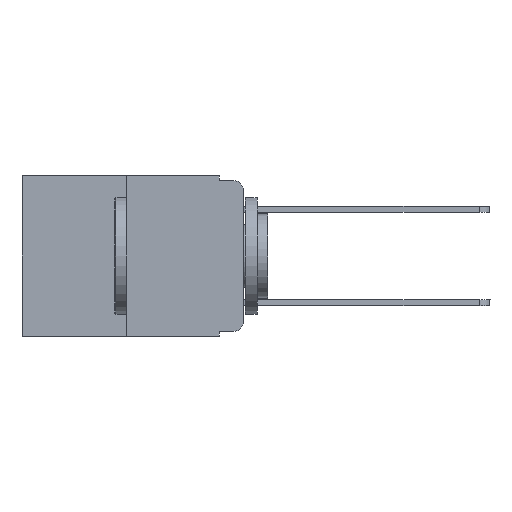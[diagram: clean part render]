
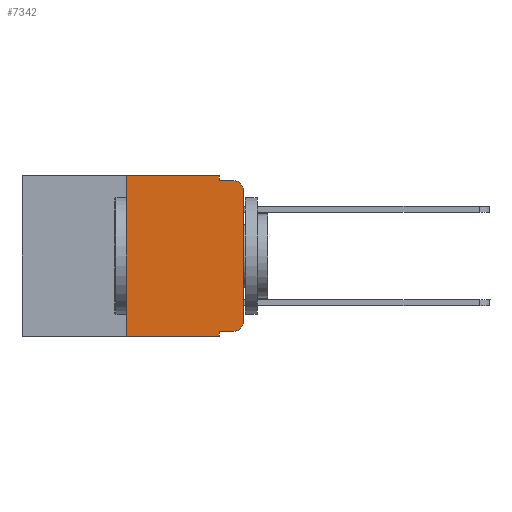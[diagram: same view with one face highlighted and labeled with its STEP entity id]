
A CAD part, left-side view. The second image highlights one B-rep face of the part: STEP entity #7342.
In plain terms, the highlighted planar face has unit normal (-1, 0, 0).
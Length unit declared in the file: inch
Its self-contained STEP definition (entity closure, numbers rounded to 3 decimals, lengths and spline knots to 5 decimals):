
#190 = CARTESIAN_POINT ( 'NONE',  ( 0., 0.02, -0.333 ) ) ;
#221 = AXIS2_PLACEMENT_3D ( 'NONE', #11391, #11540, #12854 ) ;
#326 = EDGE_CURVE ( 'NONE', #5018, #15026, #14338, .T. ) ;
#525 = DIRECTION ( 'NONE',  ( 0., 0., -1. ) ) ;
#874 = ORIENTED_EDGE ( 'NONE', *, *, #3937, .F. ) ;
#969 = ORIENTED_EDGE ( 'NONE', *, *, #7235, .T. ) ;
#1090 = CARTESIAN_POINT ( 'NONE',  ( 0., 0.051, -0.333 ) ) ;
#1106 = VECTOR ( 'NONE', #8067, 39.37008 ) ;
#1108 = ORIENTED_EDGE ( 'NONE', *, *, #9975, .T. ) ;
#1454 = EDGE_CURVE ( 'NONE', #6162, #4682, #5927, .T. ) ;
#1470 = EDGE_CURVE ( 'NONE', #2970, #7598, #14692, .T. ) ;
#1825 = CARTESIAN_POINT ( 'NONE',  ( 0., 0.051, 0. ) ) ;
#1894 = CARTESIAN_POINT ( 'NONE',  ( 0., 0., -0.313 ) ) ;
#2095 = LINE ( 'NONE', #7266, #9071 ) ;
#2244 = CIRCLE ( 'NONE', #221, 0.02 ) ;
#2262 = VECTOR ( 'NONE', #8314, 39.37008 ) ;
#2296 = EDGE_CURVE ( 'NONE', #5897, #6148, #2095, .T. ) ;
#2674 = ORIENTED_EDGE ( 'NONE', *, *, #8245, .F. ) ;
#2822 = LINE ( 'NONE', #1825, #8971 ) ;
#2970 = VERTEX_POINT ( 'NONE', #1894 ) ;
#2978 = ORIENTED_EDGE ( 'NONE', *, *, #8376, .F. ) ;
#3019 = PLANE ( 'NONE',  #7174 ) ;
#3064 = CARTESIAN_POINT ( 'NONE',  ( 0., 0.25, 0. ) ) ;
#3138 = VECTOR ( 'NONE', #14092, 39.37008 ) ;
#3145 = LINE ( 'NONE', #3064, #1106 ) ;
#3376 = CARTESIAN_POINT ( 'NONE',  ( 0., 0.051, -0.01 ) ) ;
#3489 = CARTESIAN_POINT ( 'NONE',  ( 0., 0., -0.03 ) ) ;
#3937 = EDGE_CURVE ( 'NONE', #8508, #12610, #4305, .T. ) ;
#4182 = ORIENTED_EDGE ( 'NONE', *, *, #326, .F. ) ;
#4305 = LINE ( 'NONE', #7858, #4400 ) ;
#4400 = VECTOR ( 'NONE', #14241, 39.37008 ) ;
#4682 = VERTEX_POINT ( 'NONE', #190 ) ;
#4805 = LINE ( 'NONE', #5873, #14015 ) ;
#4970 = DIRECTION ( 'NONE',  ( 0., -1., 0. ) ) ;
#5018 = VERTEX_POINT ( 'NONE', #10090 ) ;
#5476 = DIRECTION ( 'NONE',  ( 1., 0., 0. ) ) ;
#5873 = CARTESIAN_POINT ( 'NONE',  ( 0., 0.051, 0. ) ) ;
#5897 = VERTEX_POINT ( 'NONE', #8848 ) ;
#5927 = LINE ( 'NONE', #1090, #2262 ) ;
#6086 = AXIS2_PLACEMENT_3D ( 'NONE', #7183, #8176, #8341 ) ;
#6148 = VERTEX_POINT ( 'NONE', #8497 ) ;
#6162 = VERTEX_POINT ( 'NONE', #8583 ) ;
#6395 = CARTESIAN_POINT ( 'NONE',  ( 0., 0.02, -0.01 ) ) ;
#7174 = AXIS2_PLACEMENT_3D ( 'NONE', #15721, #5476, #9412 ) ;
#7183 = CARTESIAN_POINT ( 'NONE',  ( 0., 0.02, -0.03 ) ) ;
#7235 = EDGE_CURVE ( 'NONE', #4682, #2970, #2244, .T. ) ;
#7266 = CARTESIAN_POINT ( 'NONE',  ( 0., 0.473, -0.343 ) ) ;
#7342 = ADVANCED_FACE ( 'NONE', ( #13242 ), #3019, .F. ) ;
#7367 = ORIENTED_EDGE ( 'NONE', *, *, #1470, .T. ) ;
#7380 = CARTESIAN_POINT ( 'NONE',  ( 0., 0.051, 0. ) ) ;
#7598 = VERTEX_POINT ( 'NONE', #3489 ) ;
#7858 = CARTESIAN_POINT ( 'NONE',  ( 0., 0.051, -0.01 ) ) ;
#8011 = EDGE_LOOP ( 'NONE', ( #7367, #1108, #874, #2674, #4182, #2978, #10095, #13041, #8212, #969 ) ) ;
#8067 = DIRECTION ( 'NONE',  ( 0., 0., 1. ) ) ;
#8176 = DIRECTION ( 'NONE',  ( -1., 0., 0. ) ) ;
#8212 = ORIENTED_EDGE ( 'NONE', *, *, #1454, .T. ) ;
#8245 = EDGE_CURVE ( 'NONE', #15026, #8508, #2822, .T. ) ;
#8314 = DIRECTION ( 'NONE',  ( 0., -1., 0. ) ) ;
#8341 = DIRECTION ( 'NONE',  ( 0., 0., -1. ) ) ;
#8376 = EDGE_CURVE ( 'NONE', #5897, #5018, #3145, .T. ) ;
#8420 = DIRECTION ( 'NONE',  ( 0., 0., -1. ) ) ;
#8497 = CARTESIAN_POINT ( 'NONE',  ( 0., 0.051, -0.343 ) ) ;
#8508 = VERTEX_POINT ( 'NONE', #3376 ) ;
#8583 = CARTESIAN_POINT ( 'NONE',  ( 0., 0.051, -0.333 ) ) ;
#8848 = CARTESIAN_POINT ( 'NONE',  ( 0., 0.25, -0.343 ) ) ;
#8971 = VECTOR ( 'NONE', #525, 39.37008 ) ;
#9071 = VECTOR ( 'NONE', #4970, 39.37008 ) ;
#9412 = DIRECTION ( 'NONE',  ( 0., 0., -1. ) ) ;
#9975 = EDGE_CURVE ( 'NONE', #7598, #12610, #15771, .T. ) ;
#10090 = CARTESIAN_POINT ( 'NONE',  ( 0., 0.25, 0. ) ) ;
#10095 = ORIENTED_EDGE ( 'NONE', *, *, #2296, .T. ) ;
#10264 = CARTESIAN_POINT ( 'NONE',  ( 0., 0.473, 0. ) ) ;
#10772 = CARTESIAN_POINT ( 'NONE',  ( 0., 0., 0. ) ) ;
#11103 = DIRECTION ( 'NONE',  ( 0., 0., 1. ) ) ;
#11391 = CARTESIAN_POINT ( 'NONE',  ( 0., 0.02, -0.313 ) ) ;
#11427 = VECTOR ( 'NONE', #11103, 39.37008 ) ;
#11540 = DIRECTION ( 'NONE',  ( -1., 0., 0. ) ) ;
#12610 = VERTEX_POINT ( 'NONE', #6395 ) ;
#12854 = DIRECTION ( 'NONE',  ( 0., 0., -1. ) ) ;
#13041 = ORIENTED_EDGE ( 'NONE', *, *, #13328, .F. ) ;
#13242 = FACE_OUTER_BOUND ( 'NONE', #8011, .T. ) ;
#13328 = EDGE_CURVE ( 'NONE', #6162, #6148, #4805, .T. ) ;
#14015 = VECTOR ( 'NONE', #8420, 39.37008 ) ;
#14092 = DIRECTION ( 'NONE',  ( 0., -1., 0. ) ) ;
#14241 = DIRECTION ( 'NONE',  ( 0., -1., 0. ) ) ;
#14338 = LINE ( 'NONE', #10264, #3138 ) ;
#14692 = LINE ( 'NONE', #10772, #11427 ) ;
#15026 = VERTEX_POINT ( 'NONE', #7380 ) ;
#15721 = CARTESIAN_POINT ( 'NONE',  ( 0., 0.473, 0. ) ) ;
#15771 = CIRCLE ( 'NONE', #6086, 0.02 ) ;
